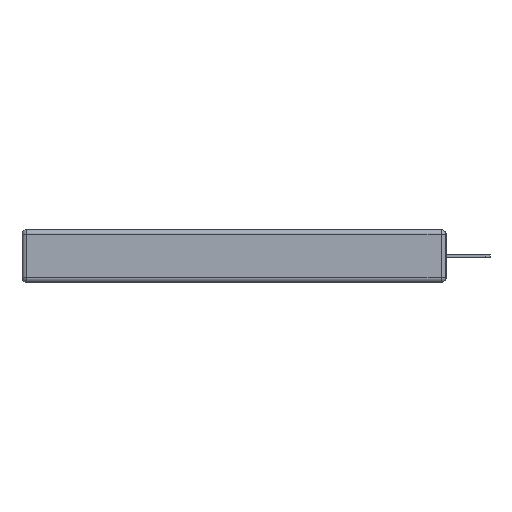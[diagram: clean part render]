
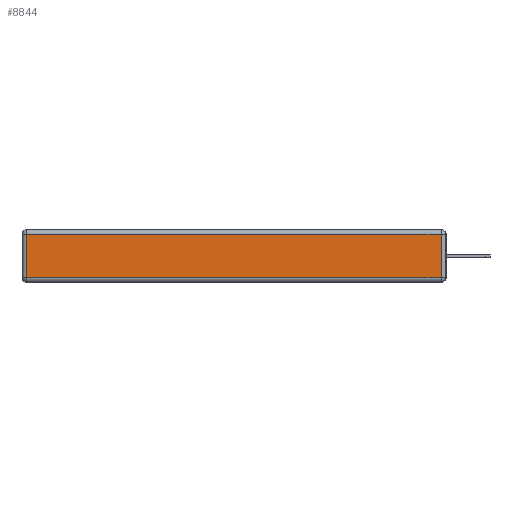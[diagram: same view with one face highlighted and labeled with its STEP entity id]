
A CAD part, left-side view. The second image highlights one B-rep face of the part: STEP entity #8844.
In plain terms, the highlighted planar face has unit normal (-1, 0, 0).
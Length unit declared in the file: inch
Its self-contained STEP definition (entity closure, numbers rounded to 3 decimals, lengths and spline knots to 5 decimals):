
#870 = CARTESIAN_POINT ( 'NONE',  ( 0., 2.75, -0.03 ) ) ;
#1978 = DIRECTION ( 'NONE',  ( 0., 0., 1. ) ) ;
#2142 = CARTESIAN_POINT ( 'NONE',  ( 0., 0., -0.343 ) ) ;
#2870 = CARTESIAN_POINT ( 'NONE',  ( 0., 0.03, -0.313 ) ) ;
#3327 = DIRECTION ( 'NONE',  ( 0., 0., 1. ) ) ;
#3333 = VECTOR ( 'NONE', #4365, 39.37008 ) ;
#4296 = AXIS2_PLACEMENT_3D ( 'NONE', #2142, #9316, #3327 ) ;
#4365 = DIRECTION ( 'NONE',  ( 0., 1., 0. ) ) ;
#4457 = DIRECTION ( 'NONE',  ( 0., 0., -1. ) ) ;
#4978 = VERTEX_POINT ( 'NONE', #5029 ) ;
#5029 = CARTESIAN_POINT ( 'NONE',  ( 0., 0.03, -0.03 ) ) ;
#5631 = VECTOR ( 'NONE', #1978, 39.37008 ) ;
#6655 = FACE_OUTER_BOUND ( 'NONE', #7849, .T. ) ;
#6733 = PLANE ( 'NONE',  #4296 ) ;
#7248 = VERTEX_POINT ( 'NONE', #12171 ) ;
#7340 = ORIENTED_EDGE ( 'NONE', *, *, #10613, .T. ) ;
#7454 = EDGE_CURVE ( 'NONE', #13298, #4978, #8005, .T. ) ;
#7849 = EDGE_LOOP ( 'NONE', ( #11858, #11775, #7340, #11210 ) ) ;
#8005 = LINE ( 'NONE', #11378, #5631 ) ;
#8026 = CARTESIAN_POINT ( 'NONE',  ( 0., 2.72, -0.343 ) ) ;
#8252 = LINE ( 'NONE', #8026, #14639 ) ;
#8844 = ADVANCED_FACE ( 'NONE', ( #6655 ), #6733, .T. ) ;
#9231 = DIRECTION ( 'NONE',  ( 0., -1., 0. ) ) ;
#9309 = EDGE_CURVE ( 'NONE', #9786, #13298, #10496, .T. ) ;
#9316 = DIRECTION ( 'NONE',  ( -1., 0., 0. ) ) ;
#9786 = VERTEX_POINT ( 'NONE', #13147 ) ;
#9840 = VECTOR ( 'NONE', #9231, 39.37008 ) ;
#10139 = EDGE_CURVE ( 'NONE', #7248, #9786, #8252, .T. ) ;
#10357 = LINE ( 'NONE', #870, #3333 ) ;
#10496 = LINE ( 'NONE', #12717, #9840 ) ;
#10613 = EDGE_CURVE ( 'NONE', #4978, #7248, #10357, .T. ) ;
#11210 = ORIENTED_EDGE ( 'NONE', *, *, #10139, .T. ) ;
#11378 = CARTESIAN_POINT ( 'NONE',  ( 0., 0.03, -0.343 ) ) ;
#11775 = ORIENTED_EDGE ( 'NONE', *, *, #7454, .T. ) ;
#11858 = ORIENTED_EDGE ( 'NONE', *, *, #9309, .T. ) ;
#12171 = CARTESIAN_POINT ( 'NONE',  ( 0., 2.72, -0.03 ) ) ;
#12717 = CARTESIAN_POINT ( 'NONE',  ( 0., 0., -0.313 ) ) ;
#13147 = CARTESIAN_POINT ( 'NONE',  ( 0., 2.72, -0.313 ) ) ;
#13298 = VERTEX_POINT ( 'NONE', #2870 ) ;
#14639 = VECTOR ( 'NONE', #4457, 39.37008 ) ;
